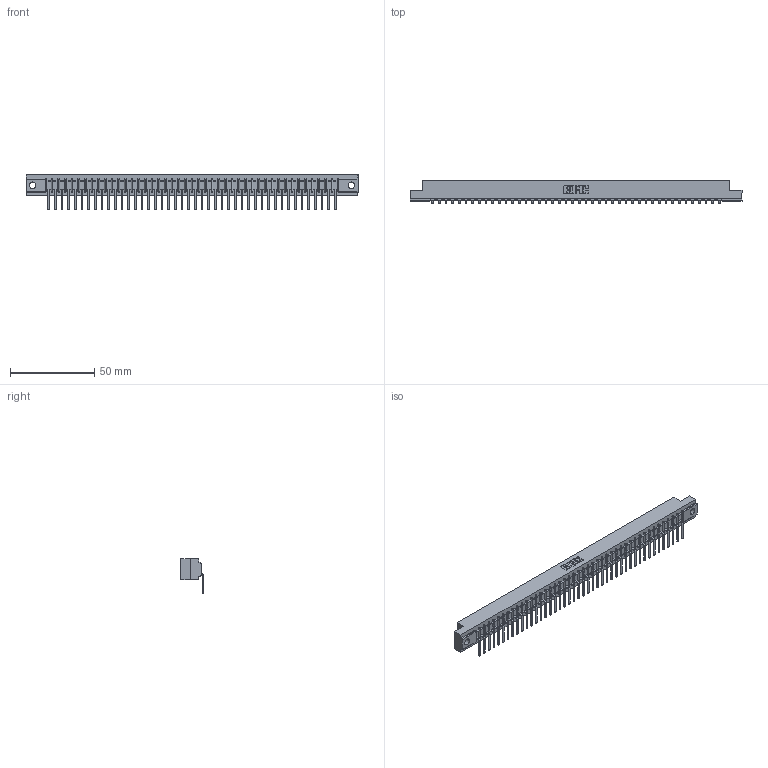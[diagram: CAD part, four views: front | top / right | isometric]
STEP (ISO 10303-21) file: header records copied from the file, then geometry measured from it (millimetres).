
FILE_DESCRIPTION (( 'STEP AP203' ), '1' );
FILE_NAME ('307-044-457-104.STEP', '2020-09-29T23:24:07', ( '' ), ( '' ), 'SwSTEP 2.0', 'SolidWorks 2020', '' );
FILE_SCHEMA (( 'CONFIG_CONTROL_DESIGN' ));
Length unit declared in the file: inch
Products named in the file (3): 307 Part_.156 Dia Mounting Holes; 307-290-002_557; 307-044-457-104
Assembly tree (45 placements, depth 2):
  307-044-457-104
    307 Part_.156 Dia Mounting Holes
    307-290-002_557  x44
Bounding box: 197.36 x 13.32 x 20.66 mm (x, y, z)
Volume: 21147.5 mm3; surface area: 27241.3 mm2
Topology: 45 solids, 45 shells, 3609 faces, 11095 edges, 7274 vertices
Faces by surface type: plane 2152, cylinder 1367, sphere 90
Entity records: 38746 total; most frequent: CARTESIAN_POINT 6542, ORIENTED_EDGE 6530, DIRECTION 6347, EDGE_CURVE 3265, VECTOR 2509, LINE 2509, VERTEX_POINT 2114, AXIS2_PLACEMENT_3D 1919
